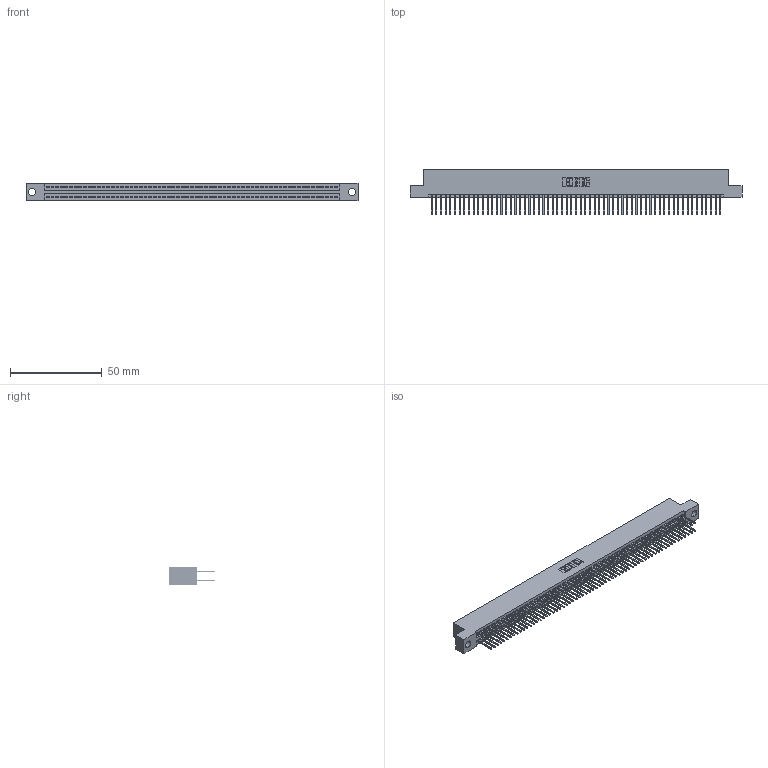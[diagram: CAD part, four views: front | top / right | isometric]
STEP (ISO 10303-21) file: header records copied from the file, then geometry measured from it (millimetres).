
FILE_DESCRIPTION (( 'STEP AP203' ), '1' );
FILE_NAME ('345-126-523-204.STEP', '2021-05-25T18:56:23', ( '' ), ( '' ), 'SwSTEP 2.0', 'SolidWorks 2020', '' );
FILE_SCHEMA (( 'CONFIG_CONTROL_DESIGN' ));
Length unit declared in the file: inch
Products named in the file (3): 345-292-001_345-293-123; 345 Part_Flush Mounting Lugs - 0.156 Dia-TI; 345-126-523-204
Assembly tree (127 placements, depth 2):
  345-126-523-204
    345 Part_Flush Mounting Lugs - 0.156 Dia-TI
    345-292-001_345-293-123  x126
Bounding box: 181.23 x 24.82 x 9.4 mm (x, y, z)
Volume: 17952 mm3; surface area: 27952.9 mm2
Topology: 127 solids, 127 shells, 6440 faces, 19151 edges, 12598 vertices
Faces by surface type: plane 4252, cylinder 2188
Entity records: 47041 total; most frequent: CARTESIAN_POINT 7870, ORIENTED_EDGE 7802, DIRECTION 6913, EDGE_CURVE 3901, VECTOR 3517, LINE 3517, VERTEX_POINT 2598, AXIS2_PLACEMENT_3D 1698
